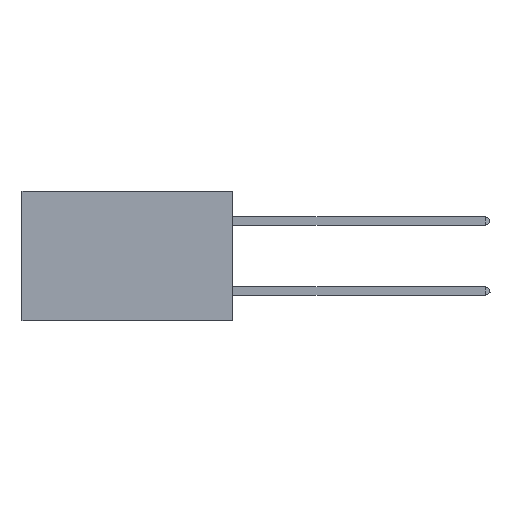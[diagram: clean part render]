
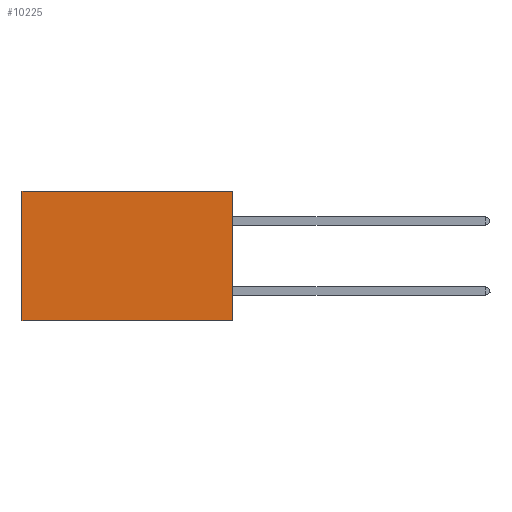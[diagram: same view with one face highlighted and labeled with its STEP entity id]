
A CAD part, left-side view. The second image highlights one B-rep face of the part: STEP entity #10225.
In plain terms, the highlighted planar face has unit normal (-1, 0, 0).
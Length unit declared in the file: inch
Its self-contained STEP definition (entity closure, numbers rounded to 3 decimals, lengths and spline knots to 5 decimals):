
#5386 = CARTESIAN_POINT ( 'NONE',  ( 0.2875, 0., 0. ) ) ;
#6551 = ORIENTED_EDGE ( 'NONE', *, *, #32048, .T. ) ;
#9002 = PLANE ( 'NONE',  #22144 ) ;
#10225 = ADVANCED_FACE ( 'NONE', ( #36951 ), #9002, .F. ) ;
#11221 = VERTEX_POINT ( 'NONE', #27773 ) ;
#12455 = DIRECTION ( 'NONE',  ( 0., 0., -1. ) ) ;
#12884 = VERTEX_POINT ( 'NONE', #35545 ) ;
#13404 = LINE ( 'NONE', #20788, #33682 ) ;
#14264 = VERTEX_POINT ( 'NONE', #42217 ) ;
#14780 = CARTESIAN_POINT ( 'NONE',  ( 0.2875, 0., -0.37 ) ) ;
#15012 = LINE ( 'NONE', #5386, #18729 ) ;
#15223 = DIRECTION ( 'NONE',  ( 0., 0., -1. ) ) ;
#15783 = EDGE_CURVE ( 'NONE', #11221, #14264, #13404, .T. ) ;
#15865 = DIRECTION ( 'NONE',  ( 1., 0., 0. ) ) ;
#18485 = ORIENTED_EDGE ( 'NONE', *, *, #36150, .F. ) ;
#18729 = VECTOR ( 'NONE', #32569, 39.37008 ) ;
#20095 = EDGE_LOOP ( 'NONE', ( #39625, #31631, #18485, #6551 ) ) ;
#20788 = CARTESIAN_POINT ( 'NONE',  ( 0.2875, 0.6, 0. ) ) ;
#22144 = AXIS2_PLACEMENT_3D ( 'NONE', #26485, #15865, #12455 ) ;
#24081 = DIRECTION ( 'NONE',  ( 0., 0., -1. ) ) ;
#24596 = EDGE_CURVE ( 'NONE', #36189, #14264, #26234, .T. ) ;
#25261 = CARTESIAN_POINT ( 'NONE',  ( 0.2875, 0., 0. ) ) ;
#26234 = LINE ( 'NONE', #28136, #28601 ) ;
#26485 = CARTESIAN_POINT ( 'NONE',  ( 0.2875, 0., 0. ) ) ;
#27773 = CARTESIAN_POINT ( 'NONE',  ( 0.2875, 0.6, 0. ) ) ;
#28083 = VECTOR ( 'NONE', #15223, 39.37008 ) ;
#28136 = CARTESIAN_POINT ( 'NONE',  ( 0.2875, 0., -0.37 ) ) ;
#28601 = VECTOR ( 'NONE', #41196, 39.37008 ) ;
#31631 = ORIENTED_EDGE ( 'NONE', *, *, #24596, .F. ) ;
#31793 = LINE ( 'NONE', #25261, #28083 ) ;
#32048 = EDGE_CURVE ( 'NONE', #12884, #11221, #15012, .T. ) ;
#32569 = DIRECTION ( 'NONE',  ( 0., 1., 0. ) ) ;
#33682 = VECTOR ( 'NONE', #24081, 39.37008 ) ;
#35545 = CARTESIAN_POINT ( 'NONE',  ( 0.2875, 0., 0. ) ) ;
#36150 = EDGE_CURVE ( 'NONE', #12884, #36189, #31793, .T. ) ;
#36189 = VERTEX_POINT ( 'NONE', #14780 ) ;
#36951 = FACE_OUTER_BOUND ( 'NONE', #20095, .T. ) ;
#39625 = ORIENTED_EDGE ( 'NONE', *, *, #15783, .T. ) ;
#41196 = DIRECTION ( 'NONE',  ( 0., 1., 0. ) ) ;
#42217 = CARTESIAN_POINT ( 'NONE',  ( 0.2875, 0.6, -0.37 ) ) ;
